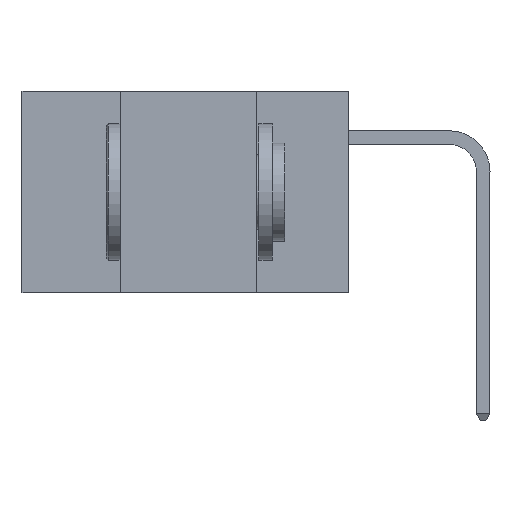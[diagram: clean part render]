
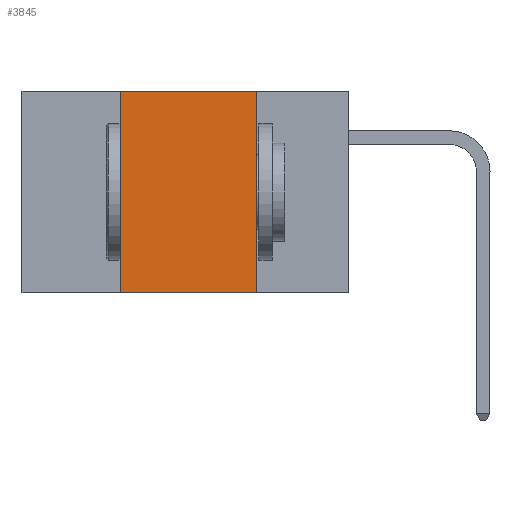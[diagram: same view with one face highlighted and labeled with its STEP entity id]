
A CAD part, left-side view. The second image highlights one B-rep face of the part: STEP entity #3845.
In plain terms, the highlighted planar face has unit normal (-1, 0, 0).
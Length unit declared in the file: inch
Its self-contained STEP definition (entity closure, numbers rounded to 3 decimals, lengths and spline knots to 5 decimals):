
#90 = AXIS2_PLACEMENT_3D ( 'NONE', #2882, #9112, #3873 ) ;
#313 = LINE ( 'NONE', #6772, #12061 ) ;
#1758 = CARTESIAN_POINT ( 'NONE',  ( 0., 0.6, 0. ) ) ;
#1867 = PLANE ( 'NONE',  #90 ) ;
#2109 = ORIENTED_EDGE ( 'NONE', *, *, #7382, .F. ) ;
#2234 = DIRECTION ( 'NONE',  ( 0., -1., 0. ) ) ;
#2405 = VERTEX_POINT ( 'NONE', #10955 ) ;
#2824 = CARTESIAN_POINT ( 'NONE',  ( 0., 0.42, 0. ) ) ;
#2854 = DIRECTION ( 'NONE',  ( 0., 0., 1. ) ) ;
#2882 = CARTESIAN_POINT ( 'NONE',  ( 0., 0.6, 0. ) ) ;
#3461 = VERTEX_POINT ( 'NONE', #7167 ) ;
#3635 = DIRECTION ( 'NONE',  ( 0., 0., -1. ) ) ;
#3845 = ADVANCED_FACE ( 'NONE', ( #6508 ), #1867, .F. ) ;
#3873 = DIRECTION ( 'NONE',  ( 0., 0., -1. ) ) ;
#4993 = ORIENTED_EDGE ( 'NONE', *, *, #5218, .F. ) ;
#5094 = LINE ( 'NONE', #8505, #7720 ) ;
#5218 = EDGE_CURVE ( 'NONE', #3461, #10801, #9555, .T. ) ;
#5534 = ORIENTED_EDGE ( 'NONE', *, *, #8578, .T. ) ;
#6377 = EDGE_CURVE ( 'NONE', #10801, #2405, #8233, .T. ) ;
#6508 = FACE_OUTER_BOUND ( 'NONE', #11543, .T. ) ;
#6772 = CARTESIAN_POINT ( 'NONE',  ( 0., 0.17, 0. ) ) ;
#7167 = CARTESIAN_POINT ( 'NONE',  ( 0., 0.42, -0.37 ) ) ;
#7382 = EDGE_CURVE ( 'NONE', #2405, #8337, #313, .T. ) ;
#7720 = VECTOR ( 'NONE', #2234, 39.37008 ) ;
#8233 = LINE ( 'NONE', #1758, #8559 ) ;
#8337 = VERTEX_POINT ( 'NONE', #12228 ) ;
#8505 = CARTESIAN_POINT ( 'NONE',  ( 0., 0.6, -0.37 ) ) ;
#8559 = VECTOR ( 'NONE', #12902, 39.37008 ) ;
#8578 = EDGE_CURVE ( 'NONE', #3461, #8337, #5094, .T. ) ;
#9112 = DIRECTION ( 'NONE',  ( 1., 0., 0. ) ) ;
#9555 = LINE ( 'NONE', #2824, #10655 ) ;
#10655 = VECTOR ( 'NONE', #2854, 39.37008 ) ;
#10801 = VERTEX_POINT ( 'NONE', #10994 ) ;
#10955 = CARTESIAN_POINT ( 'NONE',  ( 0., 0.17, 0. ) ) ;
#10994 = CARTESIAN_POINT ( 'NONE',  ( 0., 0.42, 0. ) ) ;
#11543 = EDGE_LOOP ( 'NONE', ( #2109, #11683, #4993, #5534 ) ) ;
#11683 = ORIENTED_EDGE ( 'NONE', *, *, #6377, .F. ) ;
#12061 = VECTOR ( 'NONE', #3635, 39.37008 ) ;
#12228 = CARTESIAN_POINT ( 'NONE',  ( 0., 0.17, -0.37 ) ) ;
#12902 = DIRECTION ( 'NONE',  ( 0., -1., 0. ) ) ;
